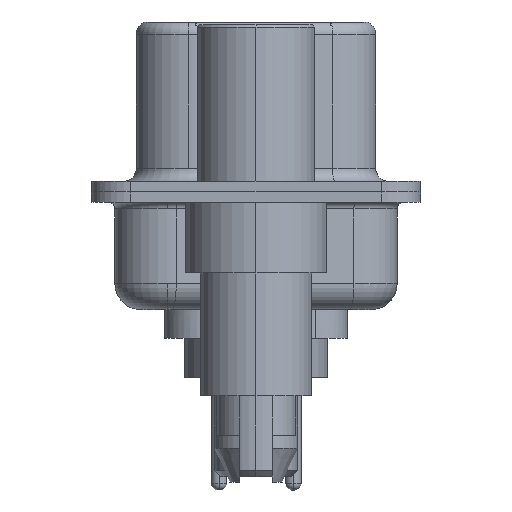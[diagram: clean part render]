
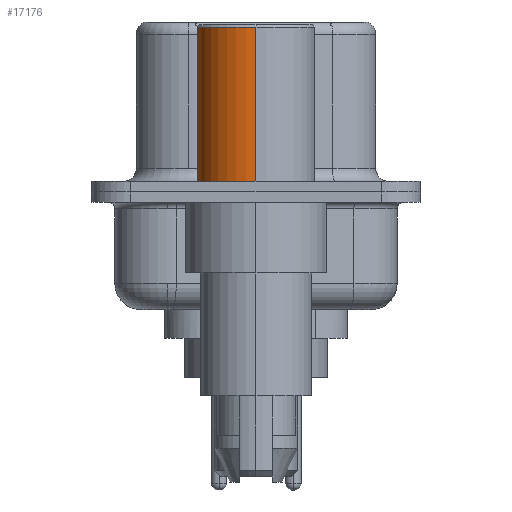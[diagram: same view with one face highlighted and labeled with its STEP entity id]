
A CAD part, left-side view. The second image highlights one B-rep face of the part: STEP entity #17176.
In plain terms, the highlighted cylindrical face has radius 2.25 mm (diameter 4.5 mm), a partial arc.
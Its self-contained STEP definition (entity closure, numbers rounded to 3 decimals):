
#247 = DIRECTION ( 'NONE',  ( 0., 0., 1. ) ) ;
#1713 = EDGE_CURVE ( 'NONE', #20407, #5069, #14556, .T. ) ;
#2445 = EDGE_LOOP ( 'NONE', ( #19116, #4290, #4124, #12802 ) ) ;
#2957 = CARTESIAN_POINT ( 'NONE',  ( -2.25, 0., 0.4 ) ) ;
#3734 = EDGE_CURVE ( 'NONE', #12375, #18571, #5024, .T. ) ;
#4096 = DIRECTION ( 'NONE',  ( 1., 0., 0. ) ) ;
#4124 = ORIENTED_EDGE ( 'NONE', *, *, #1713, .F. ) ;
#4290 = ORIENTED_EDGE ( 'NONE', *, *, #22758, .T. ) ;
#5024 = CIRCLE ( 'NONE', #5881, 2.25 ) ;
#5069 = VERTEX_POINT ( 'NONE', #8052 ) ;
#5625 = CARTESIAN_POINT ( 'NONE',  ( 2.25, 0., 0.4 ) ) ;
#5881 = AXIS2_PLACEMENT_3D ( 'NONE', #16199, #10877, #20024 ) ;
#8052 = CARTESIAN_POINT ( 'NONE',  ( -2.25, 0., 6.3 ) ) ;
#8164 = CYLINDRICAL_SURFACE ( 'NONE', #13398, 2.25 ) ;
#8374 = CARTESIAN_POINT ( 'NONE',  ( 0., 0., 6.3 ) ) ;
#8428 = DIRECTION ( 'NONE',  ( 0., 0., 1. ) ) ;
#8735 = FACE_OUTER_BOUND ( 'NONE', #2445, .T. ) ;
#9482 = DIRECTION ( 'NONE',  ( 0., 0., 1. ) ) ;
#10088 = LINE ( 'NONE', #12711, #14218 ) ;
#10877 = DIRECTION ( 'NONE',  ( 0., 0., 1. ) ) ;
#12375 = VERTEX_POINT ( 'NONE', #5625 ) ;
#12711 = CARTESIAN_POINT ( 'NONE',  ( -2.25, 0., 0.581 ) ) ;
#12802 = ORIENTED_EDGE ( 'NONE', *, *, #19691, .F. ) ;
#13398 = AXIS2_PLACEMENT_3D ( 'NONE', #16499, #9482, #4096 ) ;
#13545 = VECTOR ( 'NONE', #21239, 1000. ) ;
#13960 = DIRECTION ( 'NONE',  ( 1., 0., 0. ) ) ;
#14218 = VECTOR ( 'NONE', #247, 1000. ) ;
#14556 = CIRCLE ( 'NONE', #20110, 2.25 ) ;
#15864 = CARTESIAN_POINT ( 'NONE',  ( 2.25, 0., 0.581 ) ) ;
#16199 = CARTESIAN_POINT ( 'NONE',  ( 0., 0., 0.4 ) ) ;
#16499 = CARTESIAN_POINT ( 'NONE',  ( 0., 0., 0.581 ) ) ;
#17176 = ADVANCED_FACE ( 'NONE', ( #8735 ), #8164, .T. ) ;
#18571 = VERTEX_POINT ( 'NONE', #2957 ) ;
#18754 = LINE ( 'NONE', #15864, #13545 ) ;
#19066 = CARTESIAN_POINT ( 'NONE',  ( 2.25, 0., 6.3 ) ) ;
#19116 = ORIENTED_EDGE ( 'NONE', *, *, #3734, .T. ) ;
#19691 = EDGE_CURVE ( 'NONE', #12375, #20407, #18754, .T. ) ;
#20024 = DIRECTION ( 'NONE',  ( 1., 0., 0. ) ) ;
#20110 = AXIS2_PLACEMENT_3D ( 'NONE', #8374, #8428, #13960 ) ;
#20407 = VERTEX_POINT ( 'NONE', #19066 ) ;
#21239 = DIRECTION ( 'NONE',  ( 0., 0., 1. ) ) ;
#22758 = EDGE_CURVE ( 'NONE', #18571, #5069, #10088, .T. ) ;
